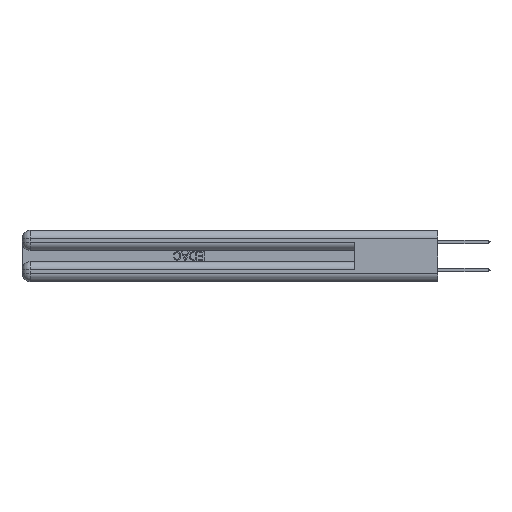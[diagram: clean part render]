
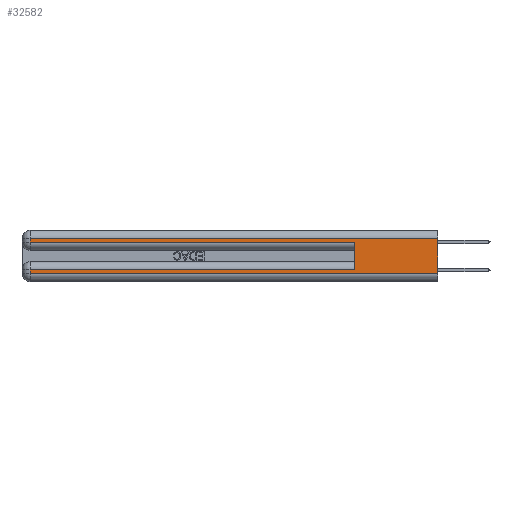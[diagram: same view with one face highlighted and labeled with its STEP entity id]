
A CAD part, left-side view. The second image highlights one B-rep face of the part: STEP entity #32582.
In plain terms, the highlighted planar face has unit normal (-1, 0, 0).
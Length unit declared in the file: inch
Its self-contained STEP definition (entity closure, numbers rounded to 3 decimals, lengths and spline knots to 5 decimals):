
#227 = VERTEX_POINT ( 'NONE', #20473 ) ;
#946 = CARTESIAN_POINT ( 'NONE',  ( 0., 0.6, 0.145 ) ) ;
#1352 = CARTESIAN_POINT ( 'NONE',  ( 0., 2.94, 0.06 ) ) ;
#1373 = VECTOR ( 'NONE', #17827, 39.37008 ) ;
#1540 = LINE ( 'NONE', #30593, #14052 ) ;
#1607 = ORIENTED_EDGE ( 'NONE', *, *, #31712, .T. ) ;
#2248 = DIRECTION ( 'NONE',  ( 0., 0., -1. ) ) ;
#3319 = ORIENTED_EDGE ( 'NONE', *, *, #28848, .T. ) ;
#5165 = ORIENTED_EDGE ( 'NONE', *, *, #41249, .T. ) ;
#6239 = VERTEX_POINT ( 'NONE', #14011 ) ;
#6446 = CARTESIAN_POINT ( 'NONE',  ( 0., 0., 0.37 ) ) ;
#6954 = DIRECTION ( 'NONE',  ( 0., 0., -1. ) ) ;
#9150 = EDGE_CURVE ( 'NONE', #227, #26070, #24121, .T. ) ;
#9607 = CARTESIAN_POINT ( 'NONE',  ( 0., 2.94, 0.37 ) ) ;
#10322 = LINE ( 'NONE', #28765, #39340 ) ;
#10418 = LINE ( 'NONE', #48632, #46649 ) ;
#10608 = VECTOR ( 'NONE', #2248, 39.37008 ) ;
#12288 = DIRECTION ( 'NONE',  ( 0., 0., 1. ) ) ;
#12721 = CARTESIAN_POINT ( 'NONE',  ( 0., 0.6, 0.285 ) ) ;
#12993 = VERTEX_POINT ( 'NONE', #22156 ) ;
#14011 = CARTESIAN_POINT ( 'NONE',  ( 0., 0., 0.06 ) ) ;
#14052 = VECTOR ( 'NONE', #30268, 39.37008 ) ;
#14628 = VECTOR ( 'NONE', #12288, 39.37008 ) ;
#14790 = VERTEX_POINT ( 'NONE', #48141 ) ;
#15267 = AXIS2_PLACEMENT_3D ( 'NONE', #6446, #29037, #6954 ) ;
#15379 = VECTOR ( 'NONE', #17305, 39.37008 ) ;
#15929 = VERTEX_POINT ( 'NONE', #20628 ) ;
#17305 = DIRECTION ( 'NONE',  ( 0., 1., 0. ) ) ;
#17827 = DIRECTION ( 'NONE',  ( 0., -1., 0. ) ) ;
#19273 = VERTEX_POINT ( 'NONE', #1352 ) ;
#19311 = CARTESIAN_POINT ( 'NONE',  ( 0., 0., 0.31 ) ) ;
#19488 = LINE ( 'NONE', #9607, #10608 ) ;
#20002 = VERTEX_POINT ( 'NONE', #34314 ) ;
#20356 = FACE_OUTER_BOUND ( 'NONE', #33170, .T. ) ;
#20473 = CARTESIAN_POINT ( 'NONE',  ( 0., 0.6, 0.085 ) ) ;
#20628 = CARTESIAN_POINT ( 'NONE',  ( 0., 2.94, 0.285 ) ) ;
#20832 = EDGE_CURVE ( 'NONE', #227, #12993, #23128, .T. ) ;
#20952 = DIRECTION ( 'NONE',  ( 0., 0., -1. ) ) ;
#22156 = CARTESIAN_POINT ( 'NONE',  ( 0., 2.94, 0.085 ) ) ;
#23128 = LINE ( 'NONE', #28948, #15379 ) ;
#24121 = LINE ( 'NONE', #946, #14628 ) ;
#24822 = ORIENTED_EDGE ( 'NONE', *, *, #36200, .T. ) ;
#25470 = CARTESIAN_POINT ( 'NONE',  ( 0., 0., 0.285 ) ) ;
#25888 = DIRECTION ( 'NONE',  ( 0., 0., -1. ) ) ;
#26070 = VERTEX_POINT ( 'NONE', #12721 ) ;
#28765 = CARTESIAN_POINT ( 'NONE',  ( 0., 2.94, 0.37 ) ) ;
#28848 = EDGE_CURVE ( 'NONE', #20002, #15929, #19488, .T. ) ;
#28948 = CARTESIAN_POINT ( 'NONE',  ( 0., 0., 0.085 ) ) ;
#29037 = DIRECTION ( 'NONE',  ( 1., 0., 0. ) ) ;
#29341 = ORIENTED_EDGE ( 'NONE', *, *, #29885, .T. ) ;
#29885 = EDGE_CURVE ( 'NONE', #19273, #6239, #1540, .T. ) ;
#30203 = LINE ( 'NONE', #19311, #33148 ) ;
#30268 = DIRECTION ( 'NONE',  ( 0., -1., 0. ) ) ;
#30408 = EDGE_CURVE ( 'NONE', #14790, #6239, #10418, .T. ) ;
#30593 = CARTESIAN_POINT ( 'NONE',  ( 0., 0., 0.06 ) ) ;
#31712 = EDGE_CURVE ( 'NONE', #12993, #19273, #10322, .T. ) ;
#31726 = LINE ( 'NONE', #25470, #1373 ) ;
#32582 = ADVANCED_FACE ( 'NONE', ( #20356 ), #40452, .F. ) ;
#33148 = VECTOR ( 'NONE', #34424, 39.37008 ) ;
#33170 = EDGE_LOOP ( 'NONE', ( #39551, #5165, #3319, #24822, #38838, #48349, #1607, #29341 ) ) ;
#34314 = CARTESIAN_POINT ( 'NONE',  ( 0., 2.94, 0.31 ) ) ;
#34424 = DIRECTION ( 'NONE',  ( 0., 1., 0. ) ) ;
#36200 = EDGE_CURVE ( 'NONE', #15929, #26070, #31726, .T. ) ;
#38838 = ORIENTED_EDGE ( 'NONE', *, *, #9150, .F. ) ;
#39340 = VECTOR ( 'NONE', #20952, 39.37008 ) ;
#39551 = ORIENTED_EDGE ( 'NONE', *, *, #30408, .F. ) ;
#40452 = PLANE ( 'NONE',  #15267 ) ;
#41249 = EDGE_CURVE ( 'NONE', #14790, #20002, #30203, .T. ) ;
#46649 = VECTOR ( 'NONE', #25888, 39.37008 ) ;
#48141 = CARTESIAN_POINT ( 'NONE',  ( 0., 0., 0.31 ) ) ;
#48349 = ORIENTED_EDGE ( 'NONE', *, *, #20832, .T. ) ;
#48632 = CARTESIAN_POINT ( 'NONE',  ( 0., 0., 0.37 ) ) ;
